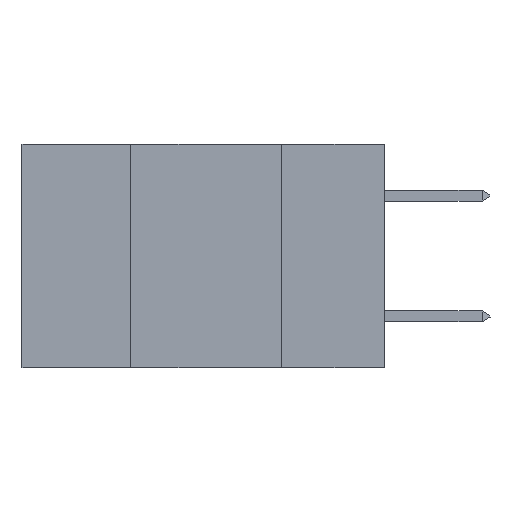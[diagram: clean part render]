
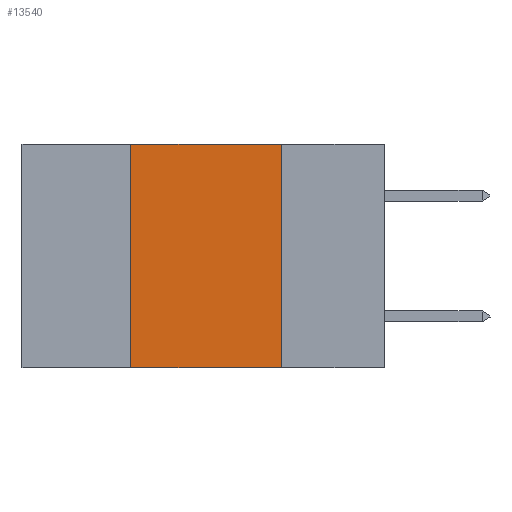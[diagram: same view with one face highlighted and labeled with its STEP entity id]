
A CAD part, left-side view. The second image highlights one B-rep face of the part: STEP entity #13540.
In plain terms, the highlighted planar face has unit normal (-1, 0, 0).
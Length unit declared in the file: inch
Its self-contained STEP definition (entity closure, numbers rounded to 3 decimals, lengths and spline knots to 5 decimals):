
#362 = ORIENTED_EDGE ( 'NONE', *, *, #4618, .F. ) ;
#537 = DIRECTION ( 'NONE',  ( 0., 0., -1. ) ) ;
#604 = DIRECTION ( 'NONE',  ( 1., 0., 0. ) ) ;
#1117 = CARTESIAN_POINT ( 'NONE',  ( 0., 0.6, -0.37 ) ) ;
#1386 = VERTEX_POINT ( 'NONE', #11514 ) ;
#2525 = VECTOR ( 'NONE', #15913, 39.37008 ) ;
#3467 = PLANE ( 'NONE',  #6134 ) ;
#3524 = LINE ( 'NONE', #8768, #3986 ) ;
#3986 = VECTOR ( 'NONE', #11565, 39.37008 ) ;
#4618 = EDGE_CURVE ( 'NONE', #13542, #17893, #3524, .T. ) ;
#5173 = VECTOR ( 'NONE', #9789, 39.37008 ) ;
#5754 = CARTESIAN_POINT ( 'NONE',  ( 0., 0.17, 0. ) ) ;
#6085 = FACE_OUTER_BOUND ( 'NONE', #12152, .T. ) ;
#6134 = AXIS2_PLACEMENT_3D ( 'NONE', #18010, #604, #537 ) ;
#6363 = LINE ( 'NONE', #16896, #10923 ) ;
#6643 = LINE ( 'NONE', #5754, #2525 ) ;
#7411 = EDGE_CURVE ( 'NONE', #17893, #15271, #6643, .T. ) ;
#7458 = ORIENTED_EDGE ( 'NONE', *, *, #17387, .T. ) ;
#7952 = CARTESIAN_POINT ( 'NONE',  ( 0., 0.17, 0. ) ) ;
#8159 = LINE ( 'NONE', #1117, #5173 ) ;
#8768 = CARTESIAN_POINT ( 'NONE',  ( 0., 0.6, 0. ) ) ;
#9248 = ORIENTED_EDGE ( 'NONE', *, *, #11176, .F. ) ;
#9789 = DIRECTION ( 'NONE',  ( 0., -1., 0. ) ) ;
#10923 = VECTOR ( 'NONE', #18380, 39.37008 ) ;
#11176 = EDGE_CURVE ( 'NONE', #1386, #13542, #6363, .T. ) ;
#11514 = CARTESIAN_POINT ( 'NONE',  ( 0., 0.42, -0.37 ) ) ;
#11565 = DIRECTION ( 'NONE',  ( 0., -1., 0. ) ) ;
#12152 = EDGE_LOOP ( 'NONE', ( #17914, #362, #9248, #7458 ) ) ;
#13540 = ADVANCED_FACE ( 'NONE', ( #6085 ), #3467, .F. ) ;
#13542 = VERTEX_POINT ( 'NONE', #17883 ) ;
#14851 = CARTESIAN_POINT ( 'NONE',  ( 0., 0.17, -0.37 ) ) ;
#15271 = VERTEX_POINT ( 'NONE', #14851 ) ;
#15913 = DIRECTION ( 'NONE',  ( 0., 0., -1. ) ) ;
#16896 = CARTESIAN_POINT ( 'NONE',  ( 0., 0.42, 0. ) ) ;
#17387 = EDGE_CURVE ( 'NONE', #1386, #15271, #8159, .T. ) ;
#17883 = CARTESIAN_POINT ( 'NONE',  ( 0., 0.42, 0. ) ) ;
#17893 = VERTEX_POINT ( 'NONE', #7952 ) ;
#17914 = ORIENTED_EDGE ( 'NONE', *, *, #7411, .F. ) ;
#18010 = CARTESIAN_POINT ( 'NONE',  ( 0., 0.6, 0. ) ) ;
#18380 = DIRECTION ( 'NONE',  ( 0., 0., 1. ) ) ;
